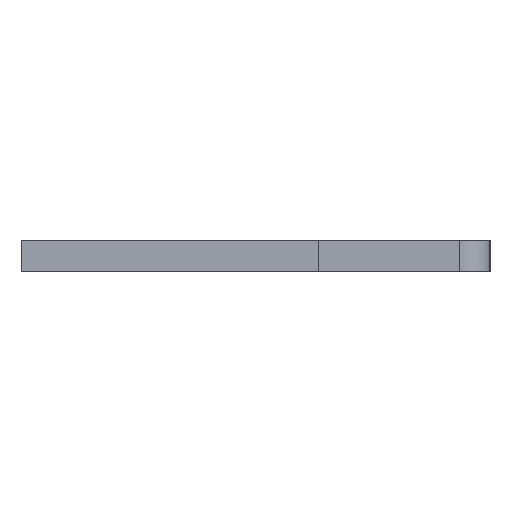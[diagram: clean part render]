
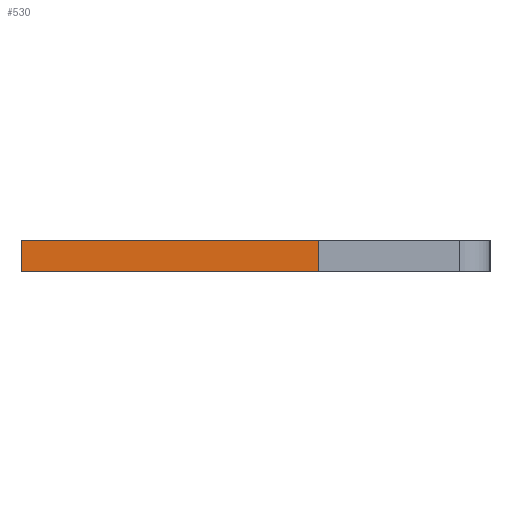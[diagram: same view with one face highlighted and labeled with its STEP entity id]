
A CAD part, left-side view. The second image highlights one B-rep face of the part: STEP entity #530.
In plain terms, the highlighted face is planar.
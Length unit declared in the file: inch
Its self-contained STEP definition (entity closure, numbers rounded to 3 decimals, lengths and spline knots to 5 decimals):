
#27 = CARTESIAN_POINT ( 'NONE',  ( -0.01, 0.15, -0.04 ) ) ;
#132 = AXIS2_PLACEMENT_3D ( 'NONE', #670, #1203, #545 ) ;
#158 = PLANE ( 'NONE',  #132 ) ;
#170 = ORIENTED_EDGE ( 'NONE', *, *, #580, .F. ) ;
#180 = DIRECTION ( 'NONE',  ( 0., 1., 0. ) ) ;
#216 = CARTESIAN_POINT ( 'NONE',  ( 0.01, 0.15, -0.04 ) ) ;
#231 = VERTEX_POINT ( 'NONE', #409 ) ;
#286 = CARTESIAN_POINT ( 'NONE',  ( 0.01, -0.04, -0.04 ) ) ;
#293 = CARTESIAN_POINT ( 'NONE',  ( -0.01, 0.15, -0.04 ) ) ;
#353 = ORIENTED_EDGE ( 'NONE', *, *, #527, .T. ) ;
#371 = LINE ( 'NONE', #27, #560 ) ;
#409 = CARTESIAN_POINT ( 'NONE',  ( -0.01, -0.04, -0.04 ) ) ;
#446 = LINE ( 'NONE', #286, #1625 ) ;
#469 = VERTEX_POINT ( 'NONE', #293 ) ;
#527 = EDGE_CURVE ( 'NONE', #891, #231, #446, .T. ) ;
#530 = ADVANCED_FACE ( 'NONE', ( #628 ), #158, .F. ) ;
#540 = DIRECTION ( 'NONE',  ( -1., 0., 0. ) ) ;
#545 = DIRECTION ( 'NONE',  ( 1., 0., 0. ) ) ;
#560 = VECTOR ( 'NONE', #180, 39.37008 ) ;
#561 = VECTOR ( 'NONE', #1529, 39.37008 ) ;
#580 = EDGE_CURVE ( 'NONE', #891, #1572, #1355, .T. ) ;
#628 = FACE_OUTER_BOUND ( 'NONE', #1124, .T. ) ;
#670 = CARTESIAN_POINT ( 'NONE',  ( 0.01, 0.15, -0.04 ) ) ;
#674 = CARTESIAN_POINT ( 'NONE',  ( 0.01, 0.15, -0.04 ) ) ;
#824 = EDGE_CURVE ( 'NONE', #1572, #469, #1006, .T. ) ;
#866 = CARTESIAN_POINT ( 'NONE',  ( 0.01, -0.04, -0.04 ) ) ;
#891 = VERTEX_POINT ( 'NONE', #866 ) ;
#908 = ORIENTED_EDGE ( 'NONE', *, *, #824, .F. ) ;
#1006 = LINE ( 'NONE', #216, #1264 ) ;
#1124 = EDGE_LOOP ( 'NONE', ( #1569, #908, #170, #353 ) ) ;
#1203 = DIRECTION ( 'NONE',  ( 0., 0., 1. ) ) ;
#1264 = VECTOR ( 'NONE', #1521, 39.37008 ) ;
#1273 = CARTESIAN_POINT ( 'NONE',  ( 0.01, 0.15, -0.04 ) ) ;
#1355 = LINE ( 'NONE', #1273, #561 ) ;
#1442 = EDGE_CURVE ( 'NONE', #231, #469, #371, .T. ) ;
#1521 = DIRECTION ( 'NONE',  ( -1., 0., 0. ) ) ;
#1529 = DIRECTION ( 'NONE',  ( 0., 1., 0. ) ) ;
#1569 = ORIENTED_EDGE ( 'NONE', *, *, #1442, .T. ) ;
#1572 = VERTEX_POINT ( 'NONE', #674 ) ;
#1625 = VECTOR ( 'NONE', #540, 39.37008 ) ;
